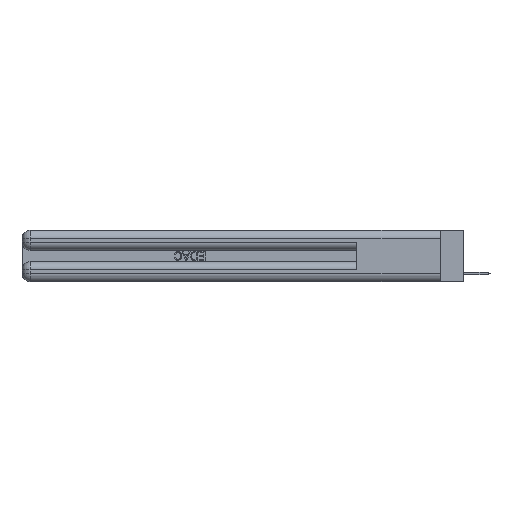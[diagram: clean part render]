
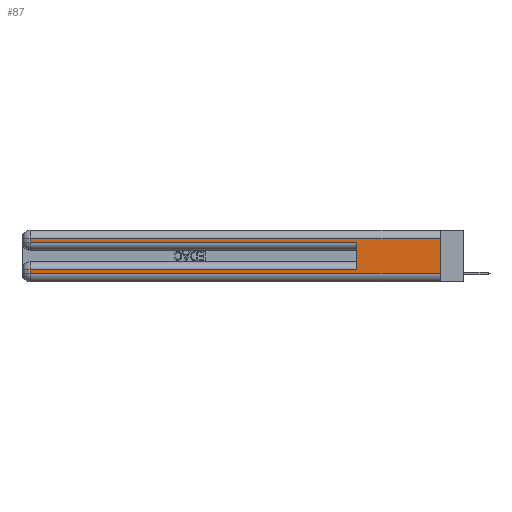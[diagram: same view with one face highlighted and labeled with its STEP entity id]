
A CAD part, left-side view. The second image highlights one B-rep face of the part: STEP entity #87.
In plain terms, the highlighted planar face has unit normal (-1, 0, 0).
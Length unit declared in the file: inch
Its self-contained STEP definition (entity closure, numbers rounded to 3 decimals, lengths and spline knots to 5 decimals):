
#87 = ADVANCED_FACE ( 'NONE', ( #17316 ), #6976, .F. ) ;
#1114 = VERTEX_POINT ( 'NONE', #23869 ) ;
#1701 = CARTESIAN_POINT ( 'NONE',  ( 0., 0., 0.285 ) ) ;
#1718 = ORIENTED_EDGE ( 'NONE', *, *, #15617, .T. ) ;
#1805 = EDGE_CURVE ( 'NONE', #10969, #21025, #6588, .T. ) ;
#1899 = CARTESIAN_POINT ( 'NONE',  ( 0., 0.6, 0.145 ) ) ;
#1970 = VECTOR ( 'NONE', #16124, 39.37008 ) ;
#2084 = CARTESIAN_POINT ( 'NONE',  ( 0., 0., 0.31 ) ) ;
#2099 = DIRECTION ( 'NONE',  ( 0., 0., 1. ) ) ;
#2184 = DIRECTION ( 'NONE',  ( 0., 1., 0. ) ) ;
#2396 = DIRECTION ( 'NONE',  ( 0., 0., -1. ) ) ;
#2934 = CARTESIAN_POINT ( 'NONE',  ( 0., 0., 0.06 ) ) ;
#2944 = LINE ( 'NONE', #4638, #21637 ) ;
#3246 = DIRECTION ( 'NONE',  ( 0., 1., 0. ) ) ;
#3278 = ORIENTED_EDGE ( 'NONE', *, *, #1805, .T. ) ;
#3471 = VECTOR ( 'NONE', #19665, 39.37008 ) ;
#3983 = ORIENTED_EDGE ( 'NONE', *, *, #8748, .T. ) ;
#4243 = DIRECTION ( 'NONE',  ( 1., 0., 0. ) ) ;
#4385 = CARTESIAN_POINT ( 'NONE',  ( 0., 0., 0.37 ) ) ;
#4638 = CARTESIAN_POINT ( 'NONE',  ( 0., 0., 0.37 ) ) ;
#5008 = LINE ( 'NONE', #2934, #19478 ) ;
#5211 = EDGE_CURVE ( 'NONE', #5932, #8796, #8138, .T. ) ;
#5582 = ORIENTED_EDGE ( 'NONE', *, *, #21270, .T. ) ;
#5932 = VERTEX_POINT ( 'NONE', #23600 ) ;
#6417 = EDGE_LOOP ( 'NONE', ( #25854, #1718, #21865, #3278, #21090, #14099, #3983, #5582 ) ) ;
#6588 = LINE ( 'NONE', #1701, #1970 ) ;
#6976 = PLANE ( 'NONE',  #7830 ) ;
#7830 = AXIS2_PLACEMENT_3D ( 'NONE', #4385, #4243, #15119 ) ;
#8138 = LINE ( 'NONE', #15855, #18352 ) ;
#8748 = EDGE_CURVE ( 'NONE', #8796, #1114, #15510, .T. ) ;
#8796 = VERTEX_POINT ( 'NONE', #11408 ) ;
#8996 = DIRECTION ( 'NONE',  ( 0., 0., -1. ) ) ;
#9010 = LINE ( 'NONE', #2084, #18184 ) ;
#9124 = EDGE_CURVE ( 'NONE', #5932, #21025, #18119, .T. ) ;
#9478 = CARTESIAN_POINT ( 'NONE',  ( 0., 2.94, 0.285 ) ) ;
#10969 = VERTEX_POINT ( 'NONE', #9478 ) ;
#11408 = CARTESIAN_POINT ( 'NONE',  ( 0., 2.94, 0.085 ) ) ;
#12392 = LINE ( 'NONE', #17707, #3471 ) ;
#12554 = VECTOR ( 'NONE', #2099, 39.37008 ) ;
#13403 = DIRECTION ( 'NONE',  ( 0., -1., 0. ) ) ;
#14099 = ORIENTED_EDGE ( 'NONE', *, *, #5211, .T. ) ;
#14257 = CARTESIAN_POINT ( 'NONE',  ( 0., 0.6, 0.285 ) ) ;
#15119 = DIRECTION ( 'NONE',  ( 0., 0., -1. ) ) ;
#15510 = LINE ( 'NONE', #25364, #26889 ) ;
#15617 = EDGE_CURVE ( 'NONE', #26364, #19047, #9010, .T. ) ;
#15855 = CARTESIAN_POINT ( 'NONE',  ( 0., 0., 0.085 ) ) ;
#16124 = DIRECTION ( 'NONE',  ( 0., -1., 0. ) ) ;
#16403 = CARTESIAN_POINT ( 'NONE',  ( 0., 0., 0.06 ) ) ;
#17316 = FACE_OUTER_BOUND ( 'NONE', #6417, .T. ) ;
#17707 = CARTESIAN_POINT ( 'NONE',  ( 0., 2.94, 0.37 ) ) ;
#18119 = LINE ( 'NONE', #1899, #12554 ) ;
#18184 = VECTOR ( 'NONE', #2184, 39.37008 ) ;
#18352 = VECTOR ( 'NONE', #3246, 39.37008 ) ;
#19047 = VERTEX_POINT ( 'NONE', #25062 ) ;
#19098 = EDGE_CURVE ( 'NONE', #19047, #10969, #12392, .T. ) ;
#19255 = EDGE_CURVE ( 'NONE', #26364, #25164, #2944, .T. ) ;
#19478 = VECTOR ( 'NONE', #13403, 39.37008 ) ;
#19665 = DIRECTION ( 'NONE',  ( 0., 0., -1. ) ) ;
#20652 = CARTESIAN_POINT ( 'NONE',  ( 0., 0., 0.31 ) ) ;
#21025 = VERTEX_POINT ( 'NONE', #14257 ) ;
#21090 = ORIENTED_EDGE ( 'NONE', *, *, #9124, .F. ) ;
#21270 = EDGE_CURVE ( 'NONE', #1114, #25164, #5008, .T. ) ;
#21637 = VECTOR ( 'NONE', #8996, 39.37008 ) ;
#21865 = ORIENTED_EDGE ( 'NONE', *, *, #19098, .T. ) ;
#23600 = CARTESIAN_POINT ( 'NONE',  ( 0., 0.6, 0.085 ) ) ;
#23869 = CARTESIAN_POINT ( 'NONE',  ( 0., 2.94, 0.06 ) ) ;
#25062 = CARTESIAN_POINT ( 'NONE',  ( 0., 2.94, 0.31 ) ) ;
#25164 = VERTEX_POINT ( 'NONE', #16403 ) ;
#25364 = CARTESIAN_POINT ( 'NONE',  ( 0., 2.94, 0.37 ) ) ;
#25854 = ORIENTED_EDGE ( 'NONE', *, *, #19255, .F. ) ;
#26364 = VERTEX_POINT ( 'NONE', #20652 ) ;
#26889 = VECTOR ( 'NONE', #2396, 39.37008 ) ;
